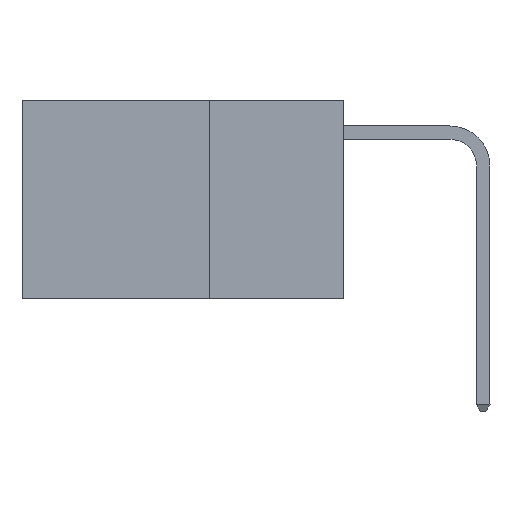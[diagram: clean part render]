
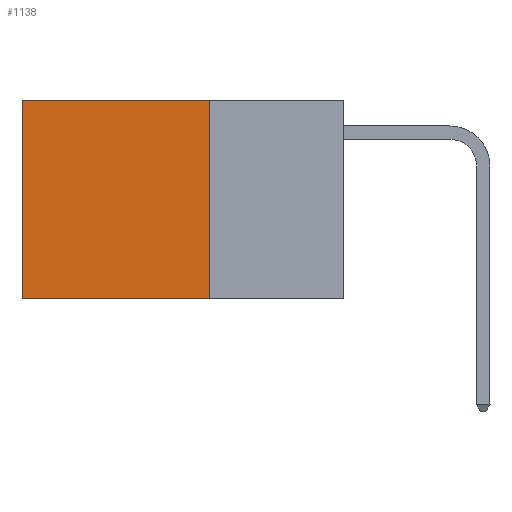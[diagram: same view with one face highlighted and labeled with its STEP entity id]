
A CAD part, left-side view. The second image highlights one B-rep face of the part: STEP entity #1138.
In plain terms, the highlighted planar face has unit normal (-1, 0, 0).
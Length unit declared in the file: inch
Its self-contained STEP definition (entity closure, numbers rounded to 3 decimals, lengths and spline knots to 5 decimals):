
#116 = VECTOR ( 'NONE', #926, 39.37008 ) ;
#193 = LINE ( 'NONE', #4151, #116 ) ;
#867 = VECTOR ( 'NONE', #3816, 39.37008 ) ;
#926 = DIRECTION ( 'NONE',  ( 0., 1., 0. ) ) ;
#1138 = ADVANCED_FACE ( 'NONE', ( #4826 ), #9629, .F. ) ;
#1149 = DIRECTION ( 'NONE',  ( 0., 0., -1. ) ) ;
#1390 = EDGE_CURVE ( 'NONE', #9976, #9146, #5113, .T. ) ;
#1630 = ORIENTED_EDGE ( 'NONE', *, *, #8203, .T. ) ;
#1906 = VERTEX_POINT ( 'NONE', #6347 ) ;
#2334 = VECTOR ( 'NONE', #7650, 39.37008 ) ;
#3203 = DIRECTION ( 'NONE',  ( 1., 0., 0. ) ) ;
#3255 = ORIENTED_EDGE ( 'NONE', *, *, #4327, .F. ) ;
#3541 = CARTESIAN_POINT ( 'NONE',  ( 0.2625, 0.25, -0.37 ) ) ;
#3780 = AXIS2_PLACEMENT_3D ( 'NONE', #5592, #3203, #1149 ) ;
#3816 = DIRECTION ( 'NONE',  ( 0., 1., 0. ) ) ;
#3930 = CARTESIAN_POINT ( 'NONE',  ( 0.2625, 0.25, 0. ) ) ;
#4095 = CARTESIAN_POINT ( 'NONE',  ( 0.2625, 0.6, -0.37 ) ) ;
#4151 = CARTESIAN_POINT ( 'NONE',  ( 0.2625, 0.25, 0. ) ) ;
#4327 = EDGE_CURVE ( 'NONE', #4560, #9976, #9543, .T. ) ;
#4489 = LINE ( 'NONE', #6734, #2334 ) ;
#4560 = VERTEX_POINT ( 'NONE', #3930 ) ;
#4826 = FACE_OUTER_BOUND ( 'NONE', #6719, .T. ) ;
#5113 = LINE ( 'NONE', #9742, #867 ) ;
#5592 = CARTESIAN_POINT ( 'NONE',  ( 0.2625, 0.25, 0. ) ) ;
#5895 = ORIENTED_EDGE ( 'NONE', *, *, #9756, .T. ) ;
#5952 = ORIENTED_EDGE ( 'NONE', *, *, #1390, .F. ) ;
#6347 = CARTESIAN_POINT ( 'NONE',  ( 0.2625, 0.6, 0. ) ) ;
#6719 = EDGE_LOOP ( 'NONE', ( #1630, #5952, #3255, #5895 ) ) ;
#6734 = CARTESIAN_POINT ( 'NONE',  ( 0.2625, 0.6, 0. ) ) ;
#7345 = VECTOR ( 'NONE', #7695, 39.37008 ) ;
#7650 = DIRECTION ( 'NONE',  ( 0., 0., -1. ) ) ;
#7695 = DIRECTION ( 'NONE',  ( 0., 0., -1. ) ) ;
#8203 = EDGE_CURVE ( 'NONE', #1906, #9146, #4489, .T. ) ;
#9136 = CARTESIAN_POINT ( 'NONE',  ( 0.2625, 0.25, 0. ) ) ;
#9146 = VERTEX_POINT ( 'NONE', #4095 ) ;
#9543 = LINE ( 'NONE', #9136, #7345 ) ;
#9629 = PLANE ( 'NONE',  #3780 ) ;
#9742 = CARTESIAN_POINT ( 'NONE',  ( 0.2625, 0.25, -0.37 ) ) ;
#9756 = EDGE_CURVE ( 'NONE', #4560, #1906, #193, .T. ) ;
#9976 = VERTEX_POINT ( 'NONE', #3541 ) ;
